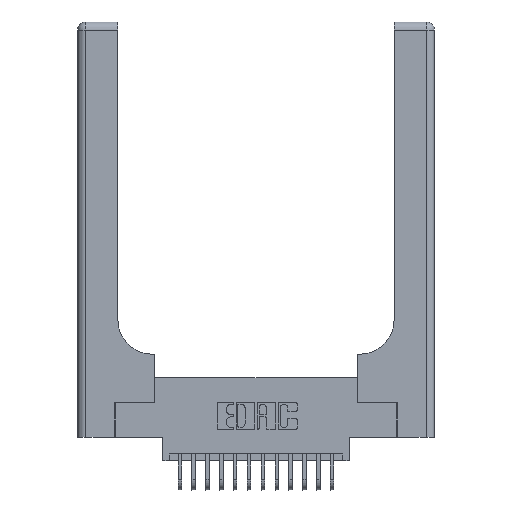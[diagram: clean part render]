
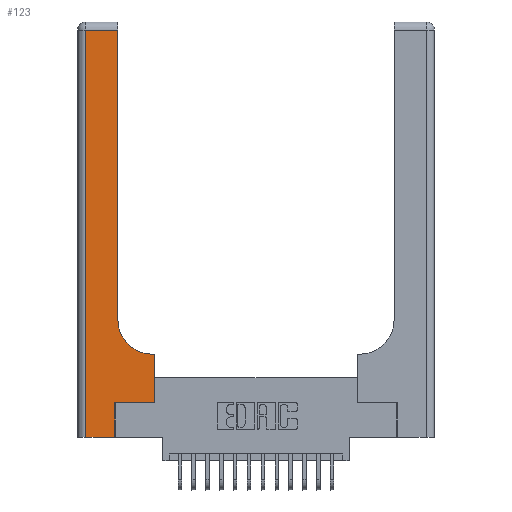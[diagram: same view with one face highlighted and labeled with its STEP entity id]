
A CAD part, top view. The second image highlights one B-rep face of the part: STEP entity #123.
In plain terms, the highlighted planar face has unit normal (0, 0, 1).
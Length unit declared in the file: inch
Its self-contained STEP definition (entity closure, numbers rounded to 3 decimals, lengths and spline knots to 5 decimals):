
#80 = ORIENTED_EDGE ( 'NONE', *, *, #10771, .T. ) ;
#123 = ADVANCED_FACE ( 'NONE', ( #1042 ), #3147, .F. ) ;
#230 = CARTESIAN_POINT ( 'NONE',  ( 0.5585, 0.6, 0.37 ) ) ;
#259 = EDGE_CURVE ( 'NONE', #13606, #2443, #8949, .T. ) ;
#1032 = CARTESIAN_POINT ( 'NONE',  ( 0.5415, 0.85, 0.37 ) ) ;
#1042 = FACE_OUTER_BOUND ( 'NONE', #9484, .T. ) ;
#1244 = LINE ( 'NONE', #10449, #3994 ) ;
#1265 = LINE ( 'NONE', #10851, #4982 ) ;
#1918 = CARTESIAN_POINT ( 'NONE',  ( 0., 0., 0.37 ) ) ;
#2443 = VERTEX_POINT ( 'NONE', #9790 ) ;
#2626 = DIRECTION ( 'NONE',  ( 0., 0., -1. ) ) ;
#2787 = ORIENTED_EDGE ( 'NONE', *, *, #15197, .T. ) ;
#2922 = DIRECTION ( 'NONE',  ( -1., 0., 0. ) ) ;
#3147 = PLANE ( 'NONE',  #9728 ) ;
#3206 = CARTESIAN_POINT ( 'NONE',  ( 0.2915, 3., 0.37 ) ) ;
#3218 = ORIENTED_EDGE ( 'NONE', *, *, #11904, .T. ) ;
#3874 = DIRECTION ( 'NONE',  ( 0., -1., 0. ) ) ;
#3994 = VECTOR ( 'NONE', #10385, 39.37008 ) ;
#4367 = LINE ( 'NONE', #6363, #16420 ) ;
#4600 = DIRECTION ( 'NONE',  ( 0., 1., 0. ) ) ;
#4982 = VECTOR ( 'NONE', #19164, 39.37008 ) ;
#5156 = ORIENTED_EDGE ( 'NONE', *, *, #12671, .T. ) ;
#5300 = CARTESIAN_POINT ( 'NONE',  ( 0.269, 0.25, 0.37 ) ) ;
#6363 = CARTESIAN_POINT ( 'NONE',  ( 0.269, 0., 0.37 ) ) ;
#7407 = DIRECTION ( 'NONE',  ( -1., 0., 0. ) ) ;
#7806 = DIRECTION ( 'NONE',  ( -1., 0., 0. ) ) ;
#8280 = CIRCLE ( 'NONE', #18857, 0.25 ) ;
#8455 = LINE ( 'NONE', #15272, #14111 ) ;
#8535 = CARTESIAN_POINT ( 'NONE',  ( 0.06, 3., 0.37 ) ) ;
#8574 = EDGE_CURVE ( 'NONE', #2443, #17166, #15018, .T. ) ;
#8836 = DIRECTION ( 'NONE',  ( 1., 0., 0. ) ) ;
#8949 = LINE ( 'NONE', #19644, #17553 ) ;
#9484 = EDGE_LOOP ( 'NONE', ( #12121, #17375, #18047, #5156, #20153, #11568, #3218, #80, #2787 ) ) ;
#9547 = VERTEX_POINT ( 'NONE', #10266 ) ;
#9728 = AXIS2_PLACEMENT_3D ( 'NONE', #15791, #15739, #7806 ) ;
#9783 = EDGE_CURVE ( 'NONE', #18812, #13606, #12507, .T. ) ;
#9790 = CARTESIAN_POINT ( 'NONE',  ( 0.06, 2.94, 0.37 ) ) ;
#9943 = CARTESIAN_POINT ( 'NONE',  ( 0.06, 0., 0.37 ) ) ;
#10266 = CARTESIAN_POINT ( 'NONE',  ( 0.5585, 0.25, 0.37 ) ) ;
#10385 = DIRECTION ( 'NONE',  ( 0., 1., 0. ) ) ;
#10449 = CARTESIAN_POINT ( 'NONE',  ( 0.5585, 0.25, 0.37 ) ) ;
#10585 = VERTEX_POINT ( 'NONE', #230 ) ;
#10771 = EDGE_CURVE ( 'NONE', #10585, #18592, #8455, .T. ) ;
#10799 = CARTESIAN_POINT ( 'NONE',  ( 0.5415, 0.6, 0.37 ) ) ;
#10851 = CARTESIAN_POINT ( 'NONE',  ( 0.269, 0.25, 0.37 ) ) ;
#11002 = VERTEX_POINT ( 'NONE', #12449 ) ;
#11357 = VECTOR ( 'NONE', #14664, 39.37008 ) ;
#11565 = VECTOR ( 'NONE', #3874, 39.37008 ) ;
#11568 = ORIENTED_EDGE ( 'NONE', *, *, #11726, .T. ) ;
#11726 = EDGE_CURVE ( 'NONE', #19951, #9547, #1265, .T. ) ;
#11904 = EDGE_CURVE ( 'NONE', #9547, #10585, #1244, .T. ) ;
#12121 = ORIENTED_EDGE ( 'NONE', *, *, #9783, .T. ) ;
#12372 = CARTESIAN_POINT ( 'NONE',  ( 0.2915, 2.94, 0.37 ) ) ;
#12449 = CARTESIAN_POINT ( 'NONE',  ( 0.269, 0., 0.37 ) ) ;
#12507 = LINE ( 'NONE', #3206, #13483 ) ;
#12576 = LINE ( 'NONE', #1918, #11357 ) ;
#12671 = EDGE_CURVE ( 'NONE', #17166, #11002, #12576, .T. ) ;
#13483 = VECTOR ( 'NONE', #4600, 39.37008 ) ;
#13606 = VERTEX_POINT ( 'NONE', #12372 ) ;
#14111 = VECTOR ( 'NONE', #7407, 39.37008 ) ;
#14664 = DIRECTION ( 'NONE',  ( 1., 0., 0. ) ) ;
#15018 = LINE ( 'NONE', #8535, #11565 ) ;
#15197 = EDGE_CURVE ( 'NONE', #18592, #18812, #8280, .T. ) ;
#15272 = CARTESIAN_POINT ( 'NONE',  ( 0.2915, 0.6, 0.37 ) ) ;
#15739 = DIRECTION ( 'NONE',  ( 0., 0., -1. ) ) ;
#15791 = CARTESIAN_POINT ( 'NONE',  ( 0., 3., 0.37 ) ) ;
#15806 = DIRECTION ( 'NONE',  ( 0., 1., 0. ) ) ;
#15868 = EDGE_CURVE ( 'NONE', #11002, #19951, #4367, .T. ) ;
#16420 = VECTOR ( 'NONE', #15806, 39.37008 ) ;
#17166 = VERTEX_POINT ( 'NONE', #9943 ) ;
#17375 = ORIENTED_EDGE ( 'NONE', *, *, #259, .T. ) ;
#17553 = VECTOR ( 'NONE', #2922, 39.37008 ) ;
#18047 = ORIENTED_EDGE ( 'NONE', *, *, #8574, .T. ) ;
#18592 = VERTEX_POINT ( 'NONE', #10799 ) ;
#18812 = VERTEX_POINT ( 'NONE', #19103 ) ;
#18857 = AXIS2_PLACEMENT_3D ( 'NONE', #1032, #2626, #8836 ) ;
#19103 = CARTESIAN_POINT ( 'NONE',  ( 0.2915, 0.85, 0.37 ) ) ;
#19164 = DIRECTION ( 'NONE',  ( 1., 0., 0. ) ) ;
#19644 = CARTESIAN_POINT ( 'NONE',  ( 0., 2.94, 0.37 ) ) ;
#19951 = VERTEX_POINT ( 'NONE', #5300 ) ;
#20153 = ORIENTED_EDGE ( 'NONE', *, *, #15868, .T. ) ;
